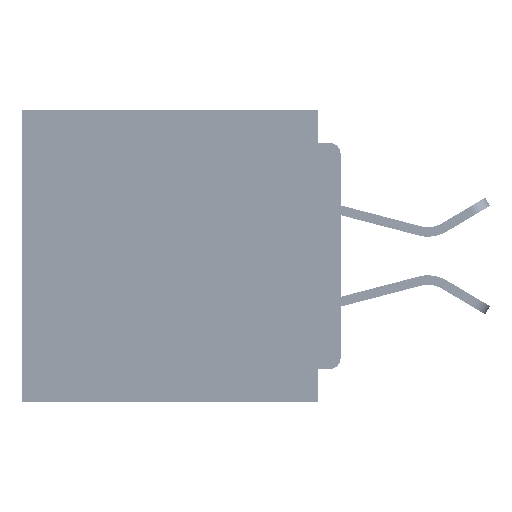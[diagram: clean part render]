
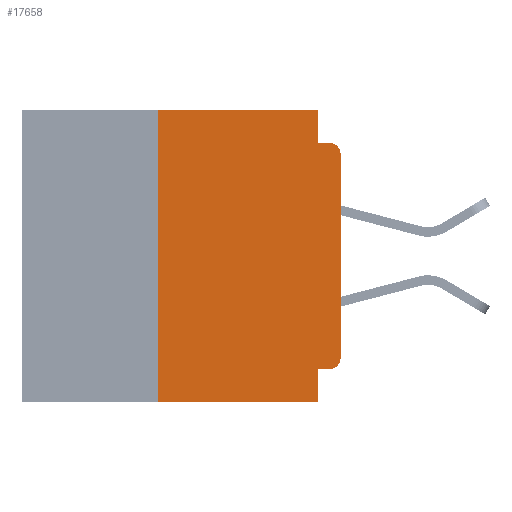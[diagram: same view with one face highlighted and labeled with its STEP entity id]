
A CAD part, left-side view. The second image highlights one B-rep face of the part: STEP entity #17658.
In plain terms, the highlighted planar face has unit normal (-1, 0, 0).
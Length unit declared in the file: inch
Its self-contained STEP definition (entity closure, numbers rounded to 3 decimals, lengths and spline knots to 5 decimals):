
#158 = DIRECTION ( 'NONE',  ( 0., -1., 0. ) ) ;
#782 = DIRECTION ( 'NONE',  ( 0., 0., -1. ) ) ;
#2471 = ORIENTED_EDGE ( 'NONE', *, *, #3262, .T. ) ;
#3262 = EDGE_CURVE ( 'NONE', #10935, #14083, #40034, .T. ) ;
#3790 = CARTESIAN_POINT ( 'NONE',  ( 0., 0.25, -0.4 ) ) ;
#3968 = CARTESIAN_POINT ( 'NONE',  ( 0., 0.437, -0.4 ) ) ;
#4897 = ORIENTED_EDGE ( 'NONE', *, *, #28387, .F. ) ;
#6728 = CARTESIAN_POINT ( 'NONE',  ( 0., 0.031, -0.355 ) ) ;
#7259 = EDGE_CURVE ( 'NONE', #22662, #33796, #8543, .T. ) ;
#8543 = LINE ( 'NONE', #14139, #39053 ) ;
#8616 = LINE ( 'NONE', #47881, #48363 ) ;
#8786 = CARTESIAN_POINT ( 'NONE',  ( 0., 0.031, -0.4 ) ) ;
#9798 = CARTESIAN_POINT ( 'NONE',  ( 0., 0.031, -0.045 ) ) ;
#9955 = CARTESIAN_POINT ( 'NONE',  ( 0., 0., -0.06 ) ) ;
#10759 = LINE ( 'NONE', #3790, #30697 ) ;
#10935 = VERTEX_POINT ( 'NONE', #26542 ) ;
#11429 = CARTESIAN_POINT ( 'NONE',  ( 0., 0.031, -0.4 ) ) ;
#12032 = LINE ( 'NONE', #31763, #33184 ) ;
#12498 = CARTESIAN_POINT ( 'NONE',  ( 0., 0.015, -0.355 ) ) ;
#12557 = EDGE_CURVE ( 'NONE', #22662, #10935, #14914, .T. ) ;
#13030 = FACE_OUTER_BOUND ( 'NONE', #18441, .T. ) ;
#13385 = ORIENTED_EDGE ( 'NONE', *, *, #28546, .F. ) ;
#13580 = AXIS2_PLACEMENT_3D ( 'NONE', #48338, #24663, #782 ) ;
#14083 = VERTEX_POINT ( 'NONE', #9955 ) ;
#14139 = CARTESIAN_POINT ( 'NONE',  ( 0., 0., -0.355 ) ) ;
#14450 = DIRECTION ( 'NONE',  ( 0., -1., 0. ) ) ;
#14711 = EDGE_CURVE ( 'NONE', #21601, #17876, #40807, .T. ) ;
#14914 = CIRCLE ( 'NONE', #13580, 0.015 ) ;
#14931 = EDGE_CURVE ( 'NONE', #22495, #39491, #10759, .T. ) ;
#15899 = DIRECTION ( 'NONE',  ( 1., 0., 0. ) ) ;
#17658 = ADVANCED_FACE ( 'NONE', ( #13030 ), #31544, .F. ) ;
#17876 = VERTEX_POINT ( 'NONE', #48656 ) ;
#18441 = EDGE_LOOP ( 'NONE', ( #2471, #27483, #40941, #4897, #39732, #46834, #20867, #13385, #41177, #36242 ) ) ;
#18504 = CARTESIAN_POINT ( 'NONE',  ( 0., 0., -0.045 ) ) ;
#19516 = DIRECTION ( 'NONE',  ( 0., 0., 1. ) ) ;
#19699 = DIRECTION ( 'NONE',  ( 0., 0., 1. ) ) ;
#20001 = DIRECTION ( 'NONE',  ( 0., 0., -1. ) ) ;
#20510 = CARTESIAN_POINT ( 'NONE',  ( 0., 0.031, 0. ) ) ;
#20816 = EDGE_CURVE ( 'NONE', #22495, #39050, #22094, .T. ) ;
#20867 = ORIENTED_EDGE ( 'NONE', *, *, #20816, .T. ) ;
#20931 = CARTESIAN_POINT ( 'NONE',  ( 0., 0.015, -0.06 ) ) ;
#21601 = VERTEX_POINT ( 'NONE', #9798 ) ;
#22094 = LINE ( 'NONE', #3968, #31358 ) ;
#22495 = VERTEX_POINT ( 'NONE', #47033 ) ;
#22662 = VERTEX_POINT ( 'NONE', #12498 ) ;
#23472 = AXIS2_PLACEMENT_3D ( 'NONE', #39719, #15899, #43679 ) ;
#24608 = EDGE_CURVE ( 'NONE', #39491, #26571, #8616, .T. ) ;
#24663 = DIRECTION ( 'NONE',  ( -1., 0., 0. ) ) ;
#24910 = DIRECTION ( 'NONE',  ( 0., 0., -1. ) ) ;
#25786 = VECTOR ( 'NONE', #44411, 39.37008 ) ;
#25900 = CARTESIAN_POINT ( 'NONE',  ( 0., 0.25, 0. ) ) ;
#26542 = CARTESIAN_POINT ( 'NONE',  ( 0., 0., -0.34 ) ) ;
#26571 = VERTEX_POINT ( 'NONE', #20510 ) ;
#27483 = ORIENTED_EDGE ( 'NONE', *, *, #36885, .T. ) ;
#27510 = CARTESIAN_POINT ( 'NONE',  ( 0., 0., 0. ) ) ;
#28387 = EDGE_CURVE ( 'NONE', #26571, #21601, #12032, .T. ) ;
#28546 = EDGE_CURVE ( 'NONE', #33796, #39050, #46780, .T. ) ;
#30159 = CIRCLE ( 'NONE', #37980, 0.015 ) ;
#30697 = VECTOR ( 'NONE', #19699, 39.37008 ) ;
#31358 = VECTOR ( 'NONE', #158, 39.37008 ) ;
#31544 = PLANE ( 'NONE',  #23472 ) ;
#31763 = CARTESIAN_POINT ( 'NONE',  ( 0., 0.031, 0. ) ) ;
#33184 = VECTOR ( 'NONE', #20001, 39.37008 ) ;
#33796 = VERTEX_POINT ( 'NONE', #6728 ) ;
#36242 = ORIENTED_EDGE ( 'NONE', *, *, #12557, .T. ) ;
#36885 = EDGE_CURVE ( 'NONE', #14083, #17876, #30159, .T. ) ;
#37980 = AXIS2_PLACEMENT_3D ( 'NONE', #20931, #48600, #24910 ) ;
#39050 = VERTEX_POINT ( 'NONE', #11429 ) ;
#39053 = VECTOR ( 'NONE', #45875, 39.37008 ) ;
#39491 = VERTEX_POINT ( 'NONE', #25900 ) ;
#39719 = CARTESIAN_POINT ( 'NONE',  ( 0., 0.437, 0. ) ) ;
#39732 = ORIENTED_EDGE ( 'NONE', *, *, #24608, .F. ) ;
#40034 = LINE ( 'NONE', #27510, #49260 ) ;
#40807 = LINE ( 'NONE', #18504, #48792 ) ;
#40941 = ORIENTED_EDGE ( 'NONE', *, *, #14711, .F. ) ;
#41177 = ORIENTED_EDGE ( 'NONE', *, *, #7259, .F. ) ;
#43679 = DIRECTION ( 'NONE',  ( 0., 0., -1. ) ) ;
#44103 = DIRECTION ( 'NONE',  ( 0., -1., 0. ) ) ;
#44411 = DIRECTION ( 'NONE',  ( 0., 0., -1. ) ) ;
#45875 = DIRECTION ( 'NONE',  ( 0., 1., 0. ) ) ;
#46780 = LINE ( 'NONE', #8786, #25786 ) ;
#46834 = ORIENTED_EDGE ( 'NONE', *, *, #14931, .F. ) ;
#47033 = CARTESIAN_POINT ( 'NONE',  ( 0., 0.25, -0.4 ) ) ;
#47881 = CARTESIAN_POINT ( 'NONE',  ( 0., 0.437, 0. ) ) ;
#48338 = CARTESIAN_POINT ( 'NONE',  ( 0., 0.015, -0.34 ) ) ;
#48363 = VECTOR ( 'NONE', #44103, 39.37008 ) ;
#48600 = DIRECTION ( 'NONE',  ( -1., 0., 0. ) ) ;
#48656 = CARTESIAN_POINT ( 'NONE',  ( 0., 0.015, -0.045 ) ) ;
#48792 = VECTOR ( 'NONE', #14450, 39.37008 ) ;
#49260 = VECTOR ( 'NONE', #19516, 39.37008 ) ;
